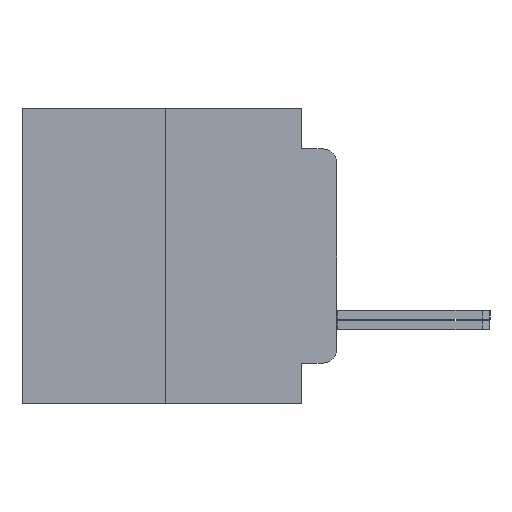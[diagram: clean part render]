
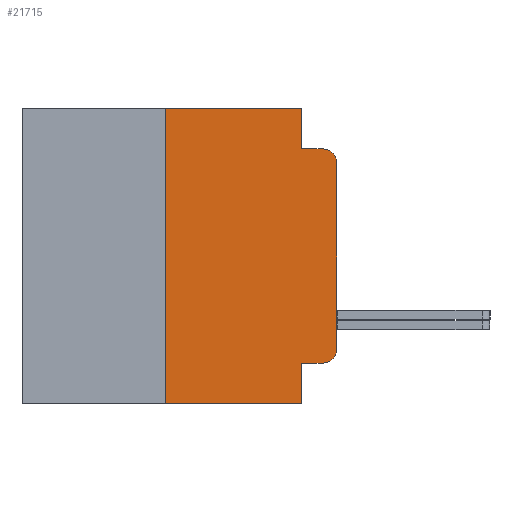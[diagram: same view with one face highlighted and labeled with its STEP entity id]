
A CAD part, left-side view. The second image highlights one B-rep face of the part: STEP entity #21715.
In plain terms, the highlighted planar face has unit normal (-1, 0, 0).
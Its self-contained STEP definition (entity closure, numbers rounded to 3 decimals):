
#306 = LINE ( 'NONE', #12389, #27762 ) ;
#831 = DIRECTION ( 'NONE',  ( 0., 0., 1. ) ) ;
#1108 = EDGE_CURVE ( 'NONE', #17587, #20664, #306, .T. ) ;
#1326 = VERTEX_POINT ( 'NONE', #18092 ) ;
#1656 = VECTOR ( 'NONE', #5738, 1000. ) ;
#2231 = CARTESIAN_POINT ( 'NONE',  ( -75.603, 1.295, -5.486 ) ) ;
#2935 = CARTESIAN_POINT ( 'NONE',  ( -75.603, 6.35, -5.486 ) ) ;
#2967 = CARTESIAN_POINT ( 'NONE',  ( -75.603, 1.295, 0. ) ) ;
#3312 = LINE ( 'NONE', #22951, #4685 ) ;
#3707 = CARTESIAN_POINT ( 'NONE',  ( -75.603, 11.684, 5.486 ) ) ;
#4165 = VERTEX_POINT ( 'NONE', #2231 ) ;
#4685 = VECTOR ( 'NONE', #12083, 1000. ) ;
#4857 = ORIENTED_EDGE ( 'NONE', *, *, #19069, .T. ) ;
#4860 = PLANE ( 'NONE',  #23939 ) ;
#5233 = EDGE_CURVE ( 'NONE', #27166, #7582, #20559, .T. ) ;
#5738 = DIRECTION ( 'NONE',  ( 0., -1., 0. ) ) ;
#6152 = EDGE_CURVE ( 'NONE', #17587, #4165, #13982, .T. ) ;
#6784 = CARTESIAN_POINT ( 'NONE',  ( -75.603, 0.508, 3.467 ) ) ;
#7582 = VERTEX_POINT ( 'NONE', #18421 ) ;
#7788 = ORIENTED_EDGE ( 'NONE', *, *, #5233, .F. ) ;
#8737 = VECTOR ( 'NONE', #831, 1000. ) ;
#8922 = VECTOR ( 'NONE', #20602, 1000. ) ;
#8968 = DIRECTION ( 'NONE',  ( 0., 0., -1. ) ) ;
#9557 = ORIENTED_EDGE ( 'NONE', *, *, #26476, .F. ) ;
#9893 = ORIENTED_EDGE ( 'NONE', *, *, #16099, .F. ) ;
#11205 = VECTOR ( 'NONE', #18533, 1000. ) ;
#11266 = DIRECTION ( 'NONE',  ( 0., 0., -1. ) ) ;
#11464 = FACE_OUTER_BOUND ( 'NONE', #20748, .T. ) ;
#11536 = ORIENTED_EDGE ( 'NONE', *, *, #14500, .T. ) ;
#11682 = CARTESIAN_POINT ( 'NONE',  ( -75.603, 1.295, 5.486 ) ) ;
#11876 = ORIENTED_EDGE ( 'NONE', *, *, #22334, .T. ) ;
#12083 = DIRECTION ( 'NONE',  ( 0., 0., 1. ) ) ;
#12389 = CARTESIAN_POINT ( 'NONE',  ( -75.603, 1.295, -3.975 ) ) ;
#13903 = ORIENTED_EDGE ( 'NONE', *, *, #16566, .T. ) ;
#13982 = LINE ( 'NONE', #28680, #27202 ) ;
#14462 = CARTESIAN_POINT ( 'NONE',  ( -75.603, 0., 3.467 ) ) ;
#14500 = EDGE_CURVE ( 'NONE', #14893, #21143, #26433, .T. ) ;
#14789 = AXIS2_PLACEMENT_3D ( 'NONE', #6784, #20038, #11266 ) ;
#14893 = VERTEX_POINT ( 'NONE', #14462 ) ;
#15379 = LINE ( 'NONE', #18422, #11205 ) ;
#15384 = DIRECTION ( 'NONE',  ( 0., 0., -1. ) ) ;
#15515 = CARTESIAN_POINT ( 'NONE',  ( -75.603, 0.508, 3.975 ) ) ;
#15887 = LINE ( 'NONE', #3707, #1656 ) ;
#15958 = VERTEX_POINT ( 'NONE', #11682 ) ;
#16099 = EDGE_CURVE ( 'NONE', #7582, #15958, #15887, .T. ) ;
#16405 = CARTESIAN_POINT ( 'NONE',  ( -75.603, 0.508, -3.975 ) ) ;
#16566 = EDGE_CURVE ( 'NONE', #27166, #4165, #21101, .T. ) ;
#17408 = CARTESIAN_POINT ( 'NONE',  ( -75.603, 1.295, -3.975 ) ) ;
#17587 = VERTEX_POINT ( 'NONE', #17408 ) ;
#18092 = CARTESIAN_POINT ( 'NONE',  ( -75.603, 0., -3.467 ) ) ;
#18359 = CARTESIAN_POINT ( 'NONE',  ( -75.603, 11.684, -5.486 ) ) ;
#18421 = CARTESIAN_POINT ( 'NONE',  ( -75.603, 6.35, 5.486 ) ) ;
#18422 = CARTESIAN_POINT ( 'NONE',  ( -75.603, 1.295, 3.975 ) ) ;
#18533 = DIRECTION ( 'NONE',  ( 0., -1., 0. ) ) ;
#18561 = CARTESIAN_POINT ( 'NONE',  ( -75.603, 0.508, -3.467 ) ) ;
#18905 = CARTESIAN_POINT ( 'NONE',  ( -75.603, 1.295, 3.975 ) ) ;
#19069 = EDGE_CURVE ( 'NONE', #1326, #14893, #3312, .T. ) ;
#19837 = AXIS2_PLACEMENT_3D ( 'NONE', #18561, #27289, #20605 ) ;
#20038 = DIRECTION ( 'NONE',  ( -1., 0., 0. ) ) ;
#20206 = EDGE_CURVE ( 'NONE', #22972, #21143, #15379, .T. ) ;
#20559 = LINE ( 'NONE', #2935, #8737 ) ;
#20602 = DIRECTION ( 'NONE',  ( 0., -1., 0. ) ) ;
#20605 = DIRECTION ( 'NONE',  ( 0., 0., -1. ) ) ;
#20664 = VERTEX_POINT ( 'NONE', #16405 ) ;
#20748 = EDGE_LOOP ( 'NONE', ( #20919, #11876, #4857, #11536, #24438, #9557, #9893, #7788, #13903, #27622 ) ) ;
#20919 = ORIENTED_EDGE ( 'NONE', *, *, #1108, .T. ) ;
#21101 = LINE ( 'NONE', #18359, #8922 ) ;
#21143 = VERTEX_POINT ( 'NONE', #15515 ) ;
#21715 = ADVANCED_FACE ( 'NONE', ( #11464 ), #4860, .F. ) ;
#22269 = CARTESIAN_POINT ( 'NONE',  ( -75.603, 11.684, 5.486 ) ) ;
#22334 = EDGE_CURVE ( 'NONE', #20664, #1326, #25018, .T. ) ;
#22951 = CARTESIAN_POINT ( 'NONE',  ( -75.603, 0., 5.486 ) ) ;
#22972 = VERTEX_POINT ( 'NONE', #18905 ) ;
#23939 = AXIS2_PLACEMENT_3D ( 'NONE', #22269, #24913, #8968 ) ;
#24438 = ORIENTED_EDGE ( 'NONE', *, *, #20206, .F. ) ;
#24913 = DIRECTION ( 'NONE',  ( 1., 0., 0. ) ) ;
#25018 = CIRCLE ( 'NONE', #19837, 0.508 ) ;
#26096 = DIRECTION ( 'NONE',  ( 0., -1., 0. ) ) ;
#26433 = CIRCLE ( 'NONE', #14789, 0.508 ) ;
#26476 = EDGE_CURVE ( 'NONE', #15958, #22972, #27239, .T. ) ;
#26889 = VECTOR ( 'NONE', #27057, 1000. ) ;
#27057 = DIRECTION ( 'NONE',  ( 0., 0., -1. ) ) ;
#27166 = VERTEX_POINT ( 'NONE', #27989 ) ;
#27202 = VECTOR ( 'NONE', #15384, 1000. ) ;
#27239 = LINE ( 'NONE', #2967, #26889 ) ;
#27289 = DIRECTION ( 'NONE',  ( -1., 0., 0. ) ) ;
#27622 = ORIENTED_EDGE ( 'NONE', *, *, #6152, .F. ) ;
#27762 = VECTOR ( 'NONE', #26096, 1000. ) ;
#27989 = CARTESIAN_POINT ( 'NONE',  ( -75.603, 6.35, -5.486 ) ) ;
#28680 = CARTESIAN_POINT ( 'NONE',  ( -75.603, 1.295, 0. ) ) ;
